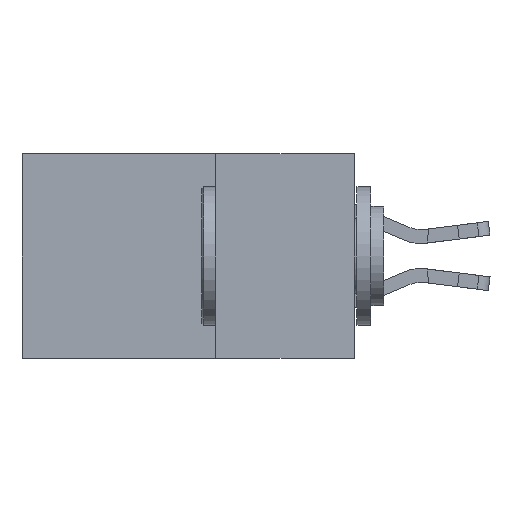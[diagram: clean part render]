
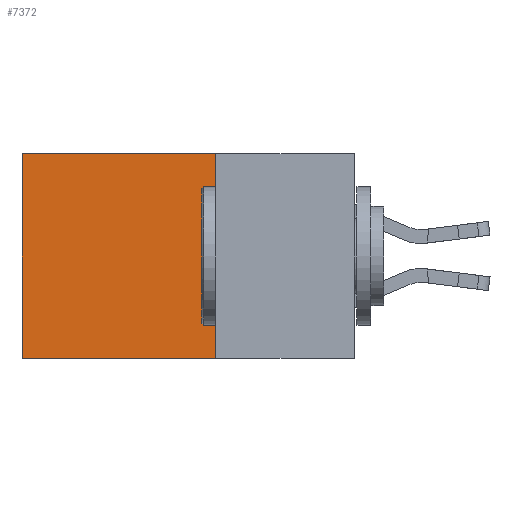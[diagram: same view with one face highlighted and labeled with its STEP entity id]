
A CAD part, left-side view. The second image highlights one B-rep face of the part: STEP entity #7372.
In plain terms, the highlighted planar face has unit normal (-1, 0, 0).
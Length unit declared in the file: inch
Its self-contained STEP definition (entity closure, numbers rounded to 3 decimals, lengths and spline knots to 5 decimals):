
#97 = ORIENTED_EDGE ( 'NONE', *, *, #5810, .T. ) ;
#133 = CARTESIAN_POINT ( 'NONE',  ( 0.2615, 0.6, -0.37 ) ) ;
#160 = VECTOR ( 'NONE', #2703, 39.37008 ) ;
#833 = CARTESIAN_POINT ( 'NONE',  ( 0.2615, 0.25, -0.37 ) ) ;
#1574 = VERTEX_POINT ( 'NONE', #833 ) ;
#1625 = CARTESIAN_POINT ( 'NONE',  ( 0.2615, 0.25, -0.37 ) ) ;
#1661 = VERTEX_POINT ( 'NONE', #5663 ) ;
#1741 = LINE ( 'NONE', #2627, #160 ) ;
#1790 = DIRECTION ( 'NONE',  ( 0., 0., -1. ) ) ;
#1833 = EDGE_CURVE ( 'NONE', #1661, #9641, #1741, .T. ) ;
#2135 = DIRECTION ( 'NONE',  ( 0., 0., -1. ) ) ;
#2627 = CARTESIAN_POINT ( 'NONE',  ( 0.2615, 0.25, 0. ) ) ;
#2703 = DIRECTION ( 'NONE',  ( 0., 1., 0. ) ) ;
#3320 = EDGE_LOOP ( 'NONE', ( #97, #6492, #3701, #3676 ) ) ;
#3673 = FACE_OUTER_BOUND ( 'NONE', #3320, .T. ) ;
#3676 = ORIENTED_EDGE ( 'NONE', *, *, #1833, .T. ) ;
#3701 = ORIENTED_EDGE ( 'NONE', *, *, #7336, .F. ) ;
#3847 = VERTEX_POINT ( 'NONE', #133 ) ;
#4418 = DIRECTION ( 'NONE',  ( 0., 0., -1. ) ) ;
#4457 = CARTESIAN_POINT ( 'NONE',  ( 0.2615, 0.25, -0.37 ) ) ;
#4488 = VECTOR ( 'NONE', #4418, 39.37008 ) ;
#4999 = LINE ( 'NONE', #1625, #4488 ) ;
#5205 = AXIS2_PLACEMENT_3D ( 'NONE', #4457, #6164, #1790 ) ;
#5663 = CARTESIAN_POINT ( 'NONE',  ( 0.2615, 0.25, 0. ) ) ;
#5810 = EDGE_CURVE ( 'NONE', #9641, #3847, #8526, .T. ) ;
#6164 = DIRECTION ( 'NONE',  ( 1., 0., 0. ) ) ;
#6238 = VECTOR ( 'NONE', #2135, 39.37008 ) ;
#6492 = ORIENTED_EDGE ( 'NONE', *, *, #10691, .F. ) ;
#6672 = DIRECTION ( 'NONE',  ( 0., 1., 0. ) ) ;
#7336 = EDGE_CURVE ( 'NONE', #1661, #1574, #4999, .T. ) ;
#7372 = ADVANCED_FACE ( 'NONE', ( #3673 ), #9455, .F. ) ;
#7424 = VECTOR ( 'NONE', #6672, 39.37008 ) ;
#8526 = LINE ( 'NONE', #8908, #6238 ) ;
#8908 = CARTESIAN_POINT ( 'NONE',  ( 0.2615, 0.6, -0.37 ) ) ;
#8909 = CARTESIAN_POINT ( 'NONE',  ( 0.2615, 0.6, 0. ) ) ;
#9455 = PLANE ( 'NONE',  #5205 ) ;
#9641 = VERTEX_POINT ( 'NONE', #8909 ) ;
#9828 = LINE ( 'NONE', #10931, #7424 ) ;
#10691 = EDGE_CURVE ( 'NONE', #1574, #3847, #9828, .T. ) ;
#10931 = CARTESIAN_POINT ( 'NONE',  ( 0.2615, 0.25, -0.37 ) ) ;
